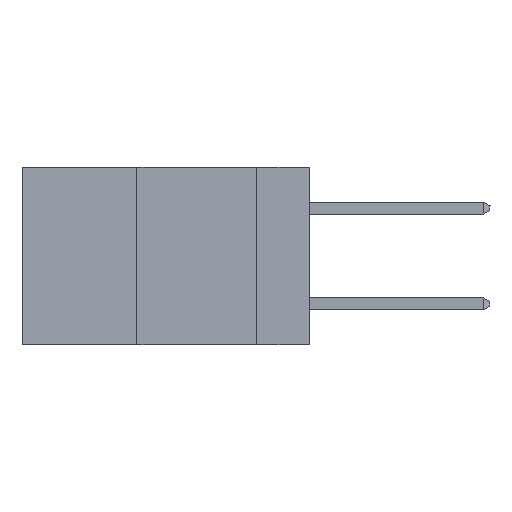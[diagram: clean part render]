
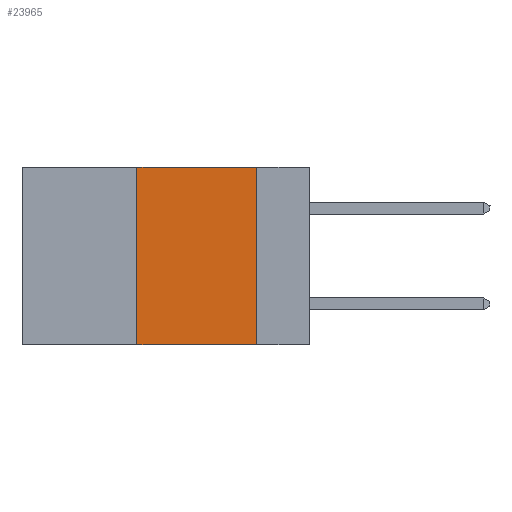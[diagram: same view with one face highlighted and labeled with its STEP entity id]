
A CAD part, left-side view. The second image highlights one B-rep face of the part: STEP entity #23965.
In plain terms, the highlighted planar face has unit normal (-1, 0, 0).
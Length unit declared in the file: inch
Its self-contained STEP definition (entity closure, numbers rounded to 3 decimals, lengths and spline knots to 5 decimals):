
#1484 = DIRECTION ( 'NONE',  ( 0., -1., 0. ) ) ;
#2146 = CARTESIAN_POINT ( 'NONE',  ( 0., 0.36, -0.37 ) ) ;
#2737 = CARTESIAN_POINT ( 'NONE',  ( 0., 0.6, 0. ) ) ;
#2775 = EDGE_LOOP ( 'NONE', ( #22139, #10652, #31004, #20806 ) ) ;
#3066 = DIRECTION ( 'NONE',  ( 1., 0., 0. ) ) ;
#3936 = CARTESIAN_POINT ( 'NONE',  ( 0., 0.6, -0.37 ) ) ;
#4401 = VECTOR ( 'NONE', #26168, 39.37008 ) ;
#5597 = CARTESIAN_POINT ( 'NONE',  ( 0., 0.36, 0. ) ) ;
#6255 = LINE ( 'NONE', #29848, #9854 ) ;
#8132 = EDGE_CURVE ( 'NONE', #17370, #28517, #6255, .T. ) ;
#8388 = CARTESIAN_POINT ( 'NONE',  ( 0., 0.11, 0. ) ) ;
#9552 = EDGE_CURVE ( 'NONE', #26578, #31631, #25349, .T. ) ;
#9854 = VECTOR ( 'NONE', #1484, 39.37008 ) ;
#10185 = LINE ( 'NONE', #18355, #19282 ) ;
#10652 = ORIENTED_EDGE ( 'NONE', *, *, #8132, .F. ) ;
#12420 = DIRECTION ( 'NONE',  ( 0., -1., 0. ) ) ;
#14514 = CARTESIAN_POINT ( 'NONE',  ( 0., 0.11, -0.37 ) ) ;
#15776 = DIRECTION ( 'NONE',  ( 0., 0., -1. ) ) ;
#17370 = VERTEX_POINT ( 'NONE', #28355 ) ;
#18355 = CARTESIAN_POINT ( 'NONE',  ( 0., 0.11, 0. ) ) ;
#19282 = VECTOR ( 'NONE', #15776, 39.37008 ) ;
#20806 = ORIENTED_EDGE ( 'NONE', *, *, #9552, .T. ) ;
#20943 = FACE_OUTER_BOUND ( 'NONE', #2775, .T. ) ;
#22139 = ORIENTED_EDGE ( 'NONE', *, *, #31009, .F. ) ;
#22393 = VECTOR ( 'NONE', #12420, 39.37008 ) ;
#23965 = ADVANCED_FACE ( 'NONE', ( #20943 ), #26188, .F. ) ;
#25349 = LINE ( 'NONE', #3936, #22393 ) ;
#26016 = DIRECTION ( 'NONE',  ( 0., 0., -1. ) ) ;
#26099 = AXIS2_PLACEMENT_3D ( 'NONE', #2737, #3066, #26016 ) ;
#26168 = DIRECTION ( 'NONE',  ( 0., 0., 1. ) ) ;
#26188 = PLANE ( 'NONE',  #26099 ) ;
#26578 = VERTEX_POINT ( 'NONE', #2146 ) ;
#28355 = CARTESIAN_POINT ( 'NONE',  ( 0., 0.36, 0. ) ) ;
#28517 = VERTEX_POINT ( 'NONE', #8388 ) ;
#28876 = LINE ( 'NONE', #5597, #4401 ) ;
#29848 = CARTESIAN_POINT ( 'NONE',  ( 0., 0.6, 0. ) ) ;
#31004 = ORIENTED_EDGE ( 'NONE', *, *, #32237, .F. ) ;
#31009 = EDGE_CURVE ( 'NONE', #28517, #31631, #10185, .T. ) ;
#31631 = VERTEX_POINT ( 'NONE', #14514 ) ;
#32237 = EDGE_CURVE ( 'NONE', #26578, #17370, #28876, .T. ) ;
